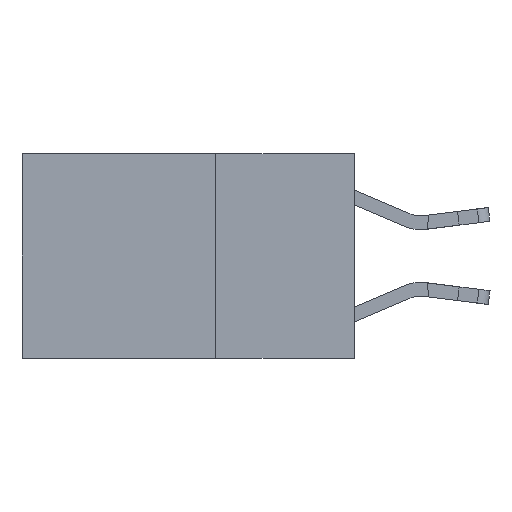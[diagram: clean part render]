
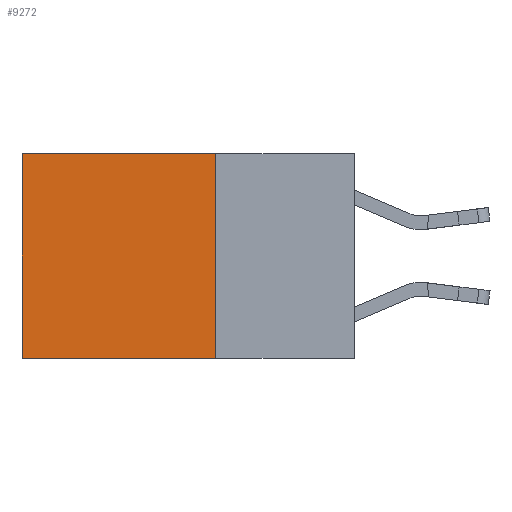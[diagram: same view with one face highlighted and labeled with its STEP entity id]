
A CAD part, left-side view. The second image highlights one B-rep face of the part: STEP entity #9272.
In plain terms, the highlighted planar face has unit normal (-1, 0, 0).
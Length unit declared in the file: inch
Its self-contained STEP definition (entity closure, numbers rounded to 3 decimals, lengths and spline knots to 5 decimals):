
#174 = EDGE_LOOP ( 'NONE', ( #10249, #4815, #4900, #8574 ) ) ;
#264 = CARTESIAN_POINT ( 'NONE',  ( 0.2625, 0.25, -0.37 ) ) ;
#285 = CARTESIAN_POINT ( 'NONE',  ( 0.2625, 0.6, 0. ) ) ;
#617 = CARTESIAN_POINT ( 'NONE',  ( 0.2625, 0.6, -0.37 ) ) ;
#898 = EDGE_CURVE ( 'NONE', #5018, #4847, #7243, .T. ) ;
#986 = AXIS2_PLACEMENT_3D ( 'NONE', #8207, #6501, #4504 ) ;
#1654 = CARTESIAN_POINT ( 'NONE',  ( 0.2625, 0.6, 0. ) ) ;
#1989 = DIRECTION ( 'NONE',  ( 0., 0., -1. ) ) ;
#3216 = DIRECTION ( 'NONE',  ( 0., 1., 0. ) ) ;
#3703 = LINE ( 'NONE', #7748, #4072 ) ;
#3804 = EDGE_CURVE ( 'NONE', #5018, #10247, #11121, .T. ) ;
#4072 = VECTOR ( 'NONE', #6805, 39.37008 ) ;
#4125 = EDGE_CURVE ( 'NONE', #10247, #10091, #3703, .T. ) ;
#4504 = DIRECTION ( 'NONE',  ( 0., 0., -1. ) ) ;
#4815 = ORIENTED_EDGE ( 'NONE', *, *, #4125, .F. ) ;
#4847 = VERTEX_POINT ( 'NONE', #1654 ) ;
#4900 = ORIENTED_EDGE ( 'NONE', *, *, #3804, .F. ) ;
#5018 = VERTEX_POINT ( 'NONE', #7215 ) ;
#6224 = CARTESIAN_POINT ( 'NONE',  ( 0.2625, 0.25, 0. ) ) ;
#6501 = DIRECTION ( 'NONE',  ( 1., 0., 0. ) ) ;
#6805 = DIRECTION ( 'NONE',  ( 0., 1., 0. ) ) ;
#7145 = EDGE_CURVE ( 'NONE', #4847, #10091, #12451, .T. ) ;
#7215 = CARTESIAN_POINT ( 'NONE',  ( 0.2625, 0.25, 0. ) ) ;
#7243 = LINE ( 'NONE', #6224, #10997 ) ;
#7748 = CARTESIAN_POINT ( 'NONE',  ( 0.2625, 0.25, -0.37 ) ) ;
#8136 = PLANE ( 'NONE',  #986 ) ;
#8207 = CARTESIAN_POINT ( 'NONE',  ( 0.2625, 0.25, 0. ) ) ;
#8262 = FACE_OUTER_BOUND ( 'NONE', #174, .T. ) ;
#8574 = ORIENTED_EDGE ( 'NONE', *, *, #898, .T. ) ;
#9122 = CARTESIAN_POINT ( 'NONE',  ( 0.2625, 0.25, 0. ) ) ;
#9272 = ADVANCED_FACE ( 'NONE', ( #8262 ), #8136, .F. ) ;
#9387 = VECTOR ( 'NONE', #1989, 39.37008 ) ;
#10091 = VERTEX_POINT ( 'NONE', #617 ) ;
#10247 = VERTEX_POINT ( 'NONE', #264 ) ;
#10249 = ORIENTED_EDGE ( 'NONE', *, *, #7145, .T. ) ;
#10324 = VECTOR ( 'NONE', #11605, 39.37008 ) ;
#10997 = VECTOR ( 'NONE', #3216, 39.37008 ) ;
#11121 = LINE ( 'NONE', #9122, #9387 ) ;
#11605 = DIRECTION ( 'NONE',  ( 0., 0., -1. ) ) ;
#12451 = LINE ( 'NONE', #285, #10324 ) ;
